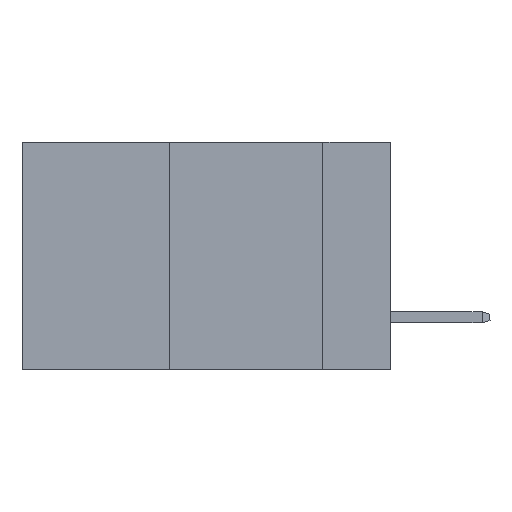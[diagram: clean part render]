
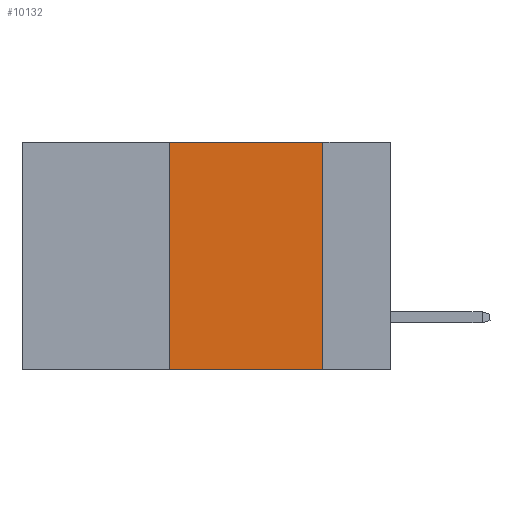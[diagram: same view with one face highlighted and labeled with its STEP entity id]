
A CAD part, left-side view. The second image highlights one B-rep face of the part: STEP entity #10132.
In plain terms, the highlighted planar face has unit normal (-1, 0, 0).
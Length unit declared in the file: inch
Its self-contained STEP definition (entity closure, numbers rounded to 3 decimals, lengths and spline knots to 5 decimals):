
#22 = VERTEX_POINT ( 'NONE', #13310 ) ;
#73 = PLANE ( 'NONE',  #15176 ) ;
#604 = CARTESIAN_POINT ( 'NONE',  ( 0., 0.11, 0. ) ) ;
#1144 = CARTESIAN_POINT ( 'NONE',  ( 0., 0.6, -0.37 ) ) ;
#1853 = VECTOR ( 'NONE', #22519, 39.37008 ) ;
#1900 = ORIENTED_EDGE ( 'NONE', *, *, #6456, .T. ) ;
#2231 = DIRECTION ( 'NONE',  ( 1., 0., 0. ) ) ;
#2846 = EDGE_LOOP ( 'NONE', ( #9697, #12621, #11315, #1900 ) ) ;
#5673 = VECTOR ( 'NONE', #9660, 39.37008 ) ;
#5701 = CARTESIAN_POINT ( 'NONE',  ( 0., 0.11, -0.37 ) ) ;
#5825 = DIRECTION ( 'NONE',  ( 0., 0., 1. ) ) ;
#6323 = LINE ( 'NONE', #19978, #5673 ) ;
#6456 = EDGE_CURVE ( 'NONE', #22, #12213, #14555, .T. ) ;
#9402 = DIRECTION ( 'NONE',  ( 0., -1., 0. ) ) ;
#9660 = DIRECTION ( 'NONE',  ( 0., 0., -1. ) ) ;
#9697 = ORIENTED_EDGE ( 'NONE', *, *, #23100, .F. ) ;
#10132 = ADVANCED_FACE ( 'NONE', ( #16105 ), #73, .F. ) ;
#10924 = VERTEX_POINT ( 'NONE', #23186 ) ;
#11015 = VECTOR ( 'NONE', #5825, 39.37008 ) ;
#11315 = ORIENTED_EDGE ( 'NONE', *, *, #13418, .F. ) ;
#12213 = VERTEX_POINT ( 'NONE', #5701 ) ;
#12621 = ORIENTED_EDGE ( 'NONE', *, *, #16016, .F. ) ;
#13310 = CARTESIAN_POINT ( 'NONE',  ( 0., 0.36, -0.37 ) ) ;
#13418 = EDGE_CURVE ( 'NONE', #22, #10924, #15908, .T. ) ;
#13908 = VECTOR ( 'NONE', #9402, 39.37008 ) ;
#14101 = CARTESIAN_POINT ( 'NONE',  ( 0., 0.36, 0. ) ) ;
#14555 = LINE ( 'NONE', #1144, #13908 ) ;
#15176 = AXIS2_PLACEMENT_3D ( 'NONE', #24941, #2231, #16758 ) ;
#15908 = LINE ( 'NONE', #14101, #11015 ) ;
#16016 = EDGE_CURVE ( 'NONE', #10924, #24141, #18394, .T. ) ;
#16105 = FACE_OUTER_BOUND ( 'NONE', #2846, .T. ) ;
#16758 = DIRECTION ( 'NONE',  ( 0., 0., -1. ) ) ;
#18394 = LINE ( 'NONE', #20418, #1853 ) ;
#19978 = CARTESIAN_POINT ( 'NONE',  ( 0., 0.11, 0. ) ) ;
#20418 = CARTESIAN_POINT ( 'NONE',  ( 0., 0.6, 0. ) ) ;
#22519 = DIRECTION ( 'NONE',  ( 0., -1., 0. ) ) ;
#23100 = EDGE_CURVE ( 'NONE', #24141, #12213, #6323, .T. ) ;
#23186 = CARTESIAN_POINT ( 'NONE',  ( 0., 0.36, 0. ) ) ;
#24141 = VERTEX_POINT ( 'NONE', #604 ) ;
#24941 = CARTESIAN_POINT ( 'NONE',  ( 0., 0.6, 0. ) ) ;
